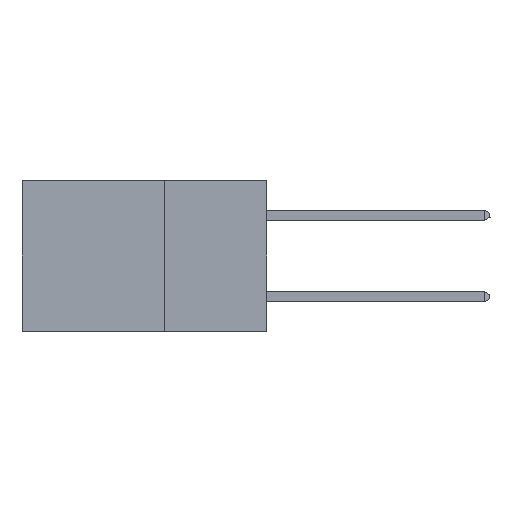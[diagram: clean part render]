
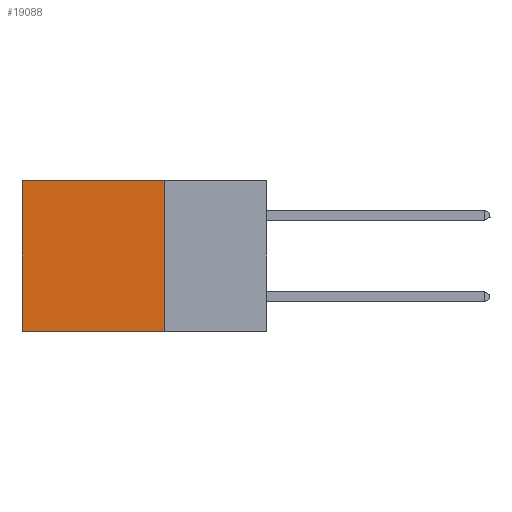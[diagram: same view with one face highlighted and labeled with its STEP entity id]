
A CAD part, left-side view. The second image highlights one B-rep face of the part: STEP entity #19088.
In plain terms, the highlighted planar face has unit normal (-1, 0, 0).
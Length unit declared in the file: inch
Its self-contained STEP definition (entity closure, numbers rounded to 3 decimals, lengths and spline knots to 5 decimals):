
#206 = CARTESIAN_POINT ( 'NONE',  ( 0.2875, 0.6, 0. ) ) ;
#1929 = EDGE_CURVE ( 'NONE', #4035, #26784, #2912, .T. ) ;
#2912 = LINE ( 'NONE', #26386, #40365 ) ;
#3113 = DIRECTION ( 'NONE',  ( 0., 1., 0. ) ) ;
#3841 = LINE ( 'NONE', #206, #8165 ) ;
#4035 = VERTEX_POINT ( 'NONE', #41161 ) ;
#5682 = DIRECTION ( 'NONE',  ( 0., 1., 0. ) ) ;
#5756 = EDGE_CURVE ( 'NONE', #35560, #26784, #3841, .T. ) ;
#8165 = VECTOR ( 'NONE', #16981, 39.37008 ) ;
#11455 = EDGE_CURVE ( 'NONE', #25968, #4035, #38240, .T. ) ;
#14684 = VECTOR ( 'NONE', #5682, 39.37008 ) ;
#14871 = FACE_OUTER_BOUND ( 'NONE', #37931, .T. ) ;
#16981 = DIRECTION ( 'NONE',  ( 0., 0., -1. ) ) ;
#19088 = ADVANCED_FACE ( 'NONE', ( #14871 ), #28005, .F. ) ;
#21674 = DIRECTION ( 'NONE',  ( 0., 0., -1. ) ) ;
#25968 = VERTEX_POINT ( 'NONE', #31281 ) ;
#26386 = CARTESIAN_POINT ( 'NONE',  ( 0.2875, 0.25, -0.37 ) ) ;
#26784 = VERTEX_POINT ( 'NONE', #28161 ) ;
#28005 = PLANE ( 'NONE',  #40214 ) ;
#28161 = CARTESIAN_POINT ( 'NONE',  ( 0.2875, 0.6, -0.37 ) ) ;
#28380 = CARTESIAN_POINT ( 'NONE',  ( 0.2875, 0.6, 0. ) ) ;
#29884 = ORIENTED_EDGE ( 'NONE', *, *, #1929, .F. ) ;
#30949 = VECTOR ( 'NONE', #21674, 39.37008 ) ;
#31281 = CARTESIAN_POINT ( 'NONE',  ( 0.2875, 0.25, 0. ) ) ;
#31884 = CARTESIAN_POINT ( 'NONE',  ( 0.2875, 0.25, 0. ) ) ;
#34196 = ORIENTED_EDGE ( 'NONE', *, *, #11455, .F. ) ;
#34909 = DIRECTION ( 'NONE',  ( 1., 0., 0. ) ) ;
#35087 = ORIENTED_EDGE ( 'NONE', *, *, #40331, .T. ) ;
#35222 = CARTESIAN_POINT ( 'NONE',  ( 0.2875, 0.25, 0. ) ) ;
#35560 = VERTEX_POINT ( 'NONE', #28380 ) ;
#37931 = EDGE_LOOP ( 'NONE', ( #38682, #29884, #34196, #35087 ) ) ;
#38240 = LINE ( 'NONE', #41678, #30949 ) ;
#38682 = ORIENTED_EDGE ( 'NONE', *, *, #5756, .T. ) ;
#39483 = LINE ( 'NONE', #35222, #14684 ) ;
#40214 = AXIS2_PLACEMENT_3D ( 'NONE', #31884, #34909, #41138 ) ;
#40331 = EDGE_CURVE ( 'NONE', #25968, #35560, #39483, .T. ) ;
#40365 = VECTOR ( 'NONE', #3113, 39.37008 ) ;
#41138 = DIRECTION ( 'NONE',  ( 0., 0., -1. ) ) ;
#41161 = CARTESIAN_POINT ( 'NONE',  ( 0.2875, 0.25, -0.37 ) ) ;
#41678 = CARTESIAN_POINT ( 'NONE',  ( 0.2875, 0.25, 0. ) ) ;
